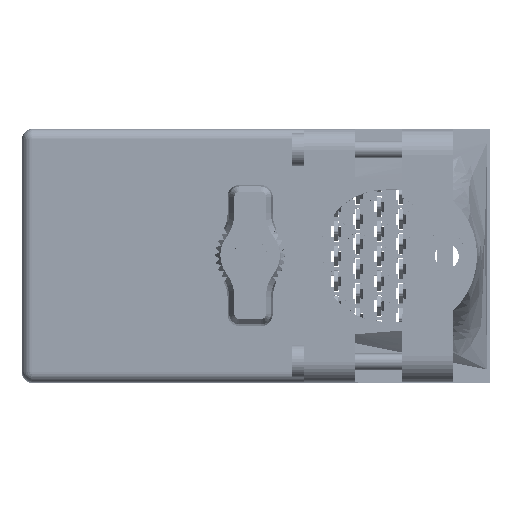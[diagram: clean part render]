
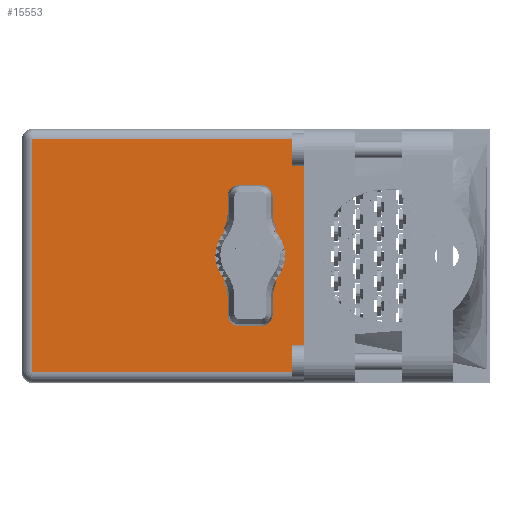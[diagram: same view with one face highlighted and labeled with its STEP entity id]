
A CAD part, top view. The second image highlights one B-rep face of the part: STEP entity #15553.
In plain terms, the highlighted face is planar.
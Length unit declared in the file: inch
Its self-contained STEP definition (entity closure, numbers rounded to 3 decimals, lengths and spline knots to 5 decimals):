
#18 = DIRECTION ( 'NONE',  ( 0., 1., 0. ) ) ;
#1092 = VERTEX_POINT ( 'NONE', #24726 ) ;
#2948 = LINE ( 'NONE', #82239, #57139 ) ;
#2986 = DIRECTION ( 'NONE',  ( 0., 1., 0. ) ) ;
#3302 = VECTOR ( 'NONE', #77506, 39.37008 ) ;
#3732 = CARTESIAN_POINT ( 'NONE',  ( 0., 2.03, -1.53 ) ) ;
#5900 = LINE ( 'NONE', #109088, #30993 ) ;
#11168 = VERTEX_POINT ( 'NONE', #36350 ) ;
#11196 = FACE_BOUND ( 'NONE', #71283, .T. ) ;
#12233 = DIRECTION ( 'NONE',  ( 0., 0., 1. ) ) ;
#15553 = ADVANCED_FACE ( 'NONE', ( #91841, #11196 ), #53616, .T. ) ;
#17375 = CARTESIAN_POINT ( 'NONE',  ( 1.705, 2.03, -0.062 ) ) ;
#17945 = ORIENTED_EDGE ( 'NONE', *, *, #34690, .F. ) ;
#18011 = CARTESIAN_POINT ( 'NONE',  ( 1.705, 2.03, -1.53 ) ) ;
#23482 = EDGE_CURVE ( 'NONE', #107921, #56267, #2948, .T. ) ;
#24285 = CARTESIAN_POINT ( 'NONE',  ( 1.705, 2.03, -1.468 ) ) ;
#24726 = CARTESIAN_POINT ( 'NONE',  ( 1.3775, 2.03, -0.8665 ) ) ;
#30966 = VERTEX_POINT ( 'NONE', #74700 ) ;
#30993 = VECTOR ( 'NONE', #92807, 39.37008 ) ;
#33871 = ORIENTED_EDGE ( 'NONE', *, *, #68392, .F. ) ;
#34690 = EDGE_CURVE ( 'NONE', #11168, #1092, #69699, .T. ) ;
#36350 = CARTESIAN_POINT ( 'NONE',  ( 1.3775, 2.03, -0.6635 ) ) ;
#41781 = DIRECTION ( 'NONE',  ( 0., 0., 1. ) ) ;
#47809 = EDGE_CURVE ( 'NONE', #75074, #30966, #66525, .T. ) ;
#48955 = EDGE_CURVE ( 'NONE', #1092, #11168, #72917, .T. ) ;
#51309 = ORIENTED_EDGE ( 'NONE', *, *, #23482, .T. ) ;
#53616 = PLANE ( 'NONE',  #79098 ) ;
#55932 = CARTESIAN_POINT ( 'NONE',  ( 1.3775, 2.03, -0.765 ) ) ;
#56262 = AXIS2_PLACEMENT_3D ( 'NONE', #55932, #89908, #56303 ) ;
#56267 = VERTEX_POINT ( 'NONE', #17375 ) ;
#56303 = DIRECTION ( 'NONE',  ( 0., 0., 1. ) ) ;
#57139 = VECTOR ( 'NONE', #108500, 39.37008 ) ;
#57297 = VECTOR ( 'NONE', #60260, 39.37008 ) ;
#60260 = DIRECTION ( 'NONE',  ( -1., 0., 0. ) ) ;
#62112 = EDGE_LOOP ( 'NONE', ( #83514, #51309, #33871, #66496 ) ) ;
#63304 = ORIENTED_EDGE ( 'NONE', *, *, #48955, .F. ) ;
#66496 = ORIENTED_EDGE ( 'NONE', *, *, #47809, .T. ) ;
#66525 = LINE ( 'NONE', #101670, #57297 ) ;
#68392 = EDGE_CURVE ( 'NONE', #75074, #56267, #87888, .T. ) ;
#69699 = CIRCLE ( 'NONE', #56262, 0.1015 ) ;
#71283 = EDGE_LOOP ( 'NONE', ( #17945, #63304 ) ) ;
#72917 = CIRCLE ( 'NONE', #109017, 0.1015 ) ;
#74700 = CARTESIAN_POINT ( 'NONE',  ( 0.062, 2.03, -1.468 ) ) ;
#75074 = VERTEX_POINT ( 'NONE', #24285 ) ;
#77506 = DIRECTION ( 'NONE',  ( 0., 0., 1. ) ) ;
#79098 = AXIS2_PLACEMENT_3D ( 'NONE', #3732, #2986, #12233 ) ;
#80476 = EDGE_CURVE ( 'NONE', #30966, #107921, #5900, .T. ) ;
#82239 = CARTESIAN_POINT ( 'NONE',  ( 1.705, 2.03, -0.062 ) ) ;
#83514 = ORIENTED_EDGE ( 'NONE', *, *, #80476, .T. ) ;
#87888 = LINE ( 'NONE', #18011, #3302 ) ;
#89908 = DIRECTION ( 'NONE',  ( 0., 1., 0. ) ) ;
#91841 = FACE_OUTER_BOUND ( 'NONE', #62112, .T. ) ;
#92401 = CARTESIAN_POINT ( 'NONE',  ( 1.3775, 2.03, -0.765 ) ) ;
#92756 = CARTESIAN_POINT ( 'NONE',  ( 0.062, 2.03, -0.062 ) ) ;
#92807 = DIRECTION ( 'NONE',  ( 0., 0., 1. ) ) ;
#101670 = CARTESIAN_POINT ( 'NONE',  ( 0., 2.03, -1.468 ) ) ;
#107921 = VERTEX_POINT ( 'NONE', #92756 ) ;
#108500 = DIRECTION ( 'NONE',  ( 1., 0., 0. ) ) ;
#109017 = AXIS2_PLACEMENT_3D ( 'NONE', #92401, #18, #41781 ) ;
#109088 = CARTESIAN_POINT ( 'NONE',  ( 0.062, 2.03, -1.53 ) ) ;
